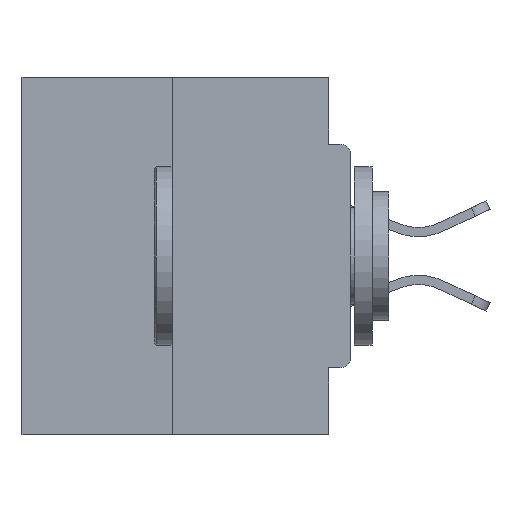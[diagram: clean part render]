
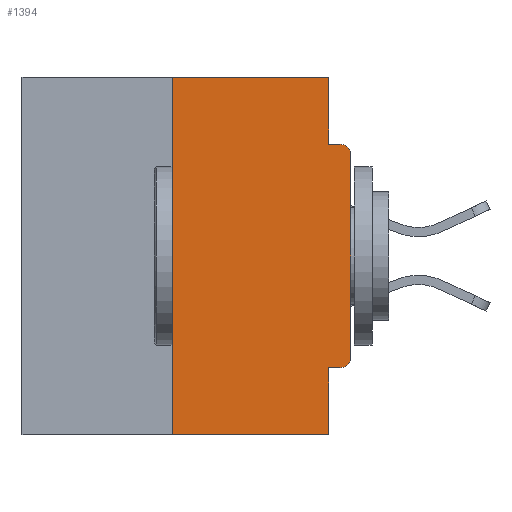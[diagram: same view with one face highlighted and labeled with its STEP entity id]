
A CAD part, left-side view. The second image highlights one B-rep face of the part: STEP entity #1394.
In plain terms, the highlighted planar face has unit normal (-1, 0, 0).
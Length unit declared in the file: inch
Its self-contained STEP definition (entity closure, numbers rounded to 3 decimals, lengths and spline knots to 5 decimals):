
#136 = EDGE_CURVE ( 'NONE', #24951, #1759, #14715, .T. ) ;
#453 = DIRECTION ( 'NONE',  ( 0., 0., -1. ) ) ;
#929 = EDGE_CURVE ( 'NONE', #4397, #10036, #26304, .T. ) ;
#1394 = ADVANCED_FACE ( 'NONE', ( #15560 ), #15247, .F. ) ;
#1509 = CARTESIAN_POINT ( 'NONE',  ( 0., 0.015, -0.4065 ) ) ;
#1579 = ORIENTED_EDGE ( 'NONE', *, *, #30736, .T. ) ;
#1601 = CARTESIAN_POINT ( 'NONE',  ( 0., 0.015, -0.0935 ) ) ;
#1759 = VERTEX_POINT ( 'NONE', #17552 ) ;
#2814 = CARTESIAN_POINT ( 'NONE',  ( 0., 0.25, -0.5 ) ) ;
#3690 = EDGE_CURVE ( 'NONE', #32830, #9355, #4913, .T. ) ;
#3752 = ORIENTED_EDGE ( 'NONE', *, *, #10531, .F. ) ;
#4397 = VERTEX_POINT ( 'NONE', #2814 ) ;
#4522 = DIRECTION ( 'NONE',  ( 0., 0., -1. ) ) ;
#4913 = CIRCLE ( 'NONE', #35515, 0.015 ) ;
#5753 = DIRECTION ( 'NONE',  ( 0., 0., -1. ) ) ;
#5940 = ORIENTED_EDGE ( 'NONE', *, *, #14226, .T. ) ;
#6126 = DIRECTION ( 'NONE',  ( 1., 0., 0. ) ) ;
#6158 = CARTESIAN_POINT ( 'NONE',  ( 0., 0.031, -0.5 ) ) ;
#6239 = CARTESIAN_POINT ( 'NONE',  ( 0., 0.031, 0. ) ) ;
#6377 = VECTOR ( 'NONE', #24348, 39.37008 ) ;
#6523 = ORIENTED_EDGE ( 'NONE', *, *, #25266, .F. ) ;
#7287 = LINE ( 'NONE', #35933, #6377 ) ;
#7531 = CARTESIAN_POINT ( 'NONE',  ( 0., 0.015, -0.3915 ) ) ;
#8036 = CARTESIAN_POINT ( 'NONE',  ( 0., 0., 0. ) ) ;
#9052 = ORIENTED_EDGE ( 'NONE', *, *, #929, .F. ) ;
#9355 = VERTEX_POINT ( 'NONE', #17240 ) ;
#10036 = VERTEX_POINT ( 'NONE', #32136 ) ;
#10273 = DIRECTION ( 'NONE',  ( -1., 0., 0. ) ) ;
#10531 = EDGE_CURVE ( 'NONE', #21352, #34743, #19613, .T. ) ;
#10665 = CARTESIAN_POINT ( 'NONE',  ( 0., 0., -0.0935 ) ) ;
#10915 = DIRECTION ( 'NONE',  ( 0., -1., 0. ) ) ;
#11094 = LINE ( 'NONE', #8036, #25439 ) ;
#11540 = VECTOR ( 'NONE', #453, 39.37008 ) ;
#11900 = VERTEX_POINT ( 'NONE', #14569 ) ;
#12329 = CARTESIAN_POINT ( 'NONE',  ( 0., 0., -0.4065 ) ) ;
#13244 = EDGE_CURVE ( 'NONE', #10036, #21352, #7287, .T. ) ;
#14226 = EDGE_CURVE ( 'NONE', #11900, #18105, #30092, .T. ) ;
#14569 = CARTESIAN_POINT ( 'NONE',  ( 0., 0., -0.1085 ) ) ;
#14715 = LINE ( 'NONE', #6158, #32655 ) ;
#14925 = ORIENTED_EDGE ( 'NONE', *, *, #16167, .F. ) ;
#15247 = PLANE ( 'NONE',  #15990 ) ;
#15560 = FACE_OUTER_BOUND ( 'NONE', #35053, .T. ) ;
#15669 = ORIENTED_EDGE ( 'NONE', *, *, #13244, .F. ) ;
#15990 = AXIS2_PLACEMENT_3D ( 'NONE', #17381, #6126, #5753 ) ;
#16167 = EDGE_CURVE ( 'NONE', #32830, #24951, #26964, .T. ) ;
#16412 = DIRECTION ( 'NONE',  ( 0., -1., 0. ) ) ;
#16925 = LINE ( 'NONE', #10665, #30856 ) ;
#17240 = CARTESIAN_POINT ( 'NONE',  ( 0., 0., -0.3915 ) ) ;
#17381 = CARTESIAN_POINT ( 'NONE',  ( 0., 0.46, 0. ) ) ;
#17552 = CARTESIAN_POINT ( 'NONE',  ( 0., 0.031, -0.5 ) ) ;
#17757 = DIRECTION ( 'NONE',  ( 0., 0., -1. ) ) ;
#17977 = VECTOR ( 'NONE', #32394, 39.37008 ) ;
#18105 = VERTEX_POINT ( 'NONE', #1601 ) ;
#19613 = LINE ( 'NONE', #6239, #11540 ) ;
#20111 = DIRECTION ( 'NONE',  ( 0., 0., -1. ) ) ;
#20346 = CARTESIAN_POINT ( 'NONE',  ( 0., 0.015, -0.1085 ) ) ;
#20766 = ORIENTED_EDGE ( 'NONE', *, *, #22159, .T. ) ;
#20811 = DIRECTION ( 'NONE',  ( 0., 0., 1. ) ) ;
#21352 = VERTEX_POINT ( 'NONE', #36579 ) ;
#21409 = AXIS2_PLACEMENT_3D ( 'NONE', #20346, #25984, #20111 ) ;
#22159 = EDGE_CURVE ( 'NONE', #4397, #1759, #33774, .T. ) ;
#22273 = VECTOR ( 'NONE', #20811, 39.37008 ) ;
#24348 = DIRECTION ( 'NONE',  ( 0., -1., 0. ) ) ;
#24951 = VERTEX_POINT ( 'NONE', #35517 ) ;
#25217 = ORIENTED_EDGE ( 'NONE', *, *, #136, .F. ) ;
#25266 = EDGE_CURVE ( 'NONE', #34743, #18105, #16925, .T. ) ;
#25439 = VECTOR ( 'NONE', #36975, 39.37008 ) ;
#25984 = DIRECTION ( 'NONE',  ( -1., 0., 0. ) ) ;
#26146 = VECTOR ( 'NONE', #10915, 39.37008 ) ;
#26304 = LINE ( 'NONE', #35246, #22273 ) ;
#26566 = ORIENTED_EDGE ( 'NONE', *, *, #3690, .T. ) ;
#26964 = LINE ( 'NONE', #12329, #17977 ) ;
#29822 = CARTESIAN_POINT ( 'NONE',  ( 0., 0.031, -0.0935 ) ) ;
#30092 = CIRCLE ( 'NONE', #21409, 0.015 ) ;
#30736 = EDGE_CURVE ( 'NONE', #9355, #11900, #11094, .T. ) ;
#30856 = VECTOR ( 'NONE', #16412, 39.37008 ) ;
#31365 = CARTESIAN_POINT ( 'NONE',  ( 0., 0.46, -0.5 ) ) ;
#32136 = CARTESIAN_POINT ( 'NONE',  ( 0., 0.25, 0. ) ) ;
#32394 = DIRECTION ( 'NONE',  ( 0., 1., 0. ) ) ;
#32655 = VECTOR ( 'NONE', #17757, 39.37008 ) ;
#32830 = VERTEX_POINT ( 'NONE', #1509 ) ;
#33774 = LINE ( 'NONE', #31365, #26146 ) ;
#34743 = VERTEX_POINT ( 'NONE', #29822 ) ;
#35053 = EDGE_LOOP ( 'NONE', ( #15669, #9052, #20766, #25217, #14925, #26566, #1579, #5940, #6523, #3752 ) ) ;
#35246 = CARTESIAN_POINT ( 'NONE',  ( 0., 0.25, 0. ) ) ;
#35515 = AXIS2_PLACEMENT_3D ( 'NONE', #7531, #10273, #4522 ) ;
#35517 = CARTESIAN_POINT ( 'NONE',  ( 0., 0.031, -0.4065 ) ) ;
#35933 = CARTESIAN_POINT ( 'NONE',  ( 0., 0.46, 0. ) ) ;
#36579 = CARTESIAN_POINT ( 'NONE',  ( 0., 0.031, 0. ) ) ;
#36975 = DIRECTION ( 'NONE',  ( 0., 0., 1. ) ) ;
